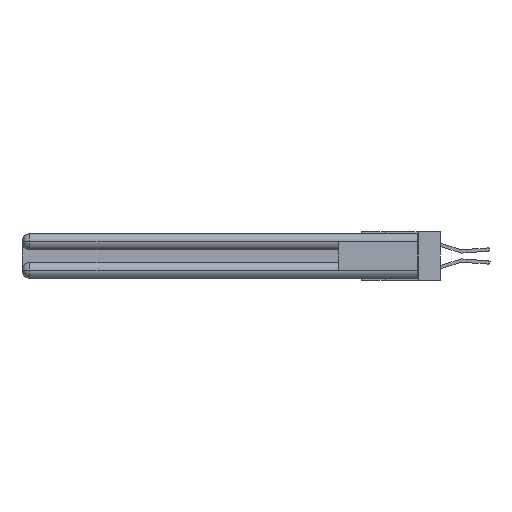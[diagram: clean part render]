
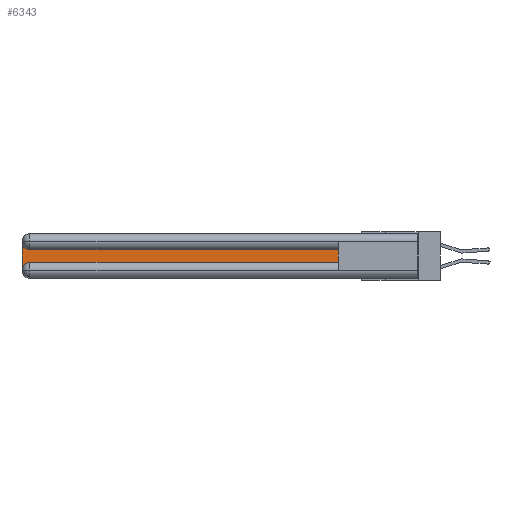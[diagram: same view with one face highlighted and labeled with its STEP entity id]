
A CAD part, left-side view. The second image highlights one B-rep face of the part: STEP entity #6343.
In plain terms, the highlighted planar face has unit normal (-1, 0, 0).
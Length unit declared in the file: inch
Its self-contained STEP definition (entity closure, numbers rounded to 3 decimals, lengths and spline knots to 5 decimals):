
#704 = ORIENTED_EDGE ( 'NONE', *, *, #27883, .T. ) ;
#1953 = LINE ( 'NONE', #17784, #20460 ) ;
#1994 = EDGE_CURVE ( 'NONE', #14123, #4935, #2353, .T. ) ;
#2238 = CARTESIAN_POINT ( 'NONE',  ( 0.075, 0.6, -0.2175 ) ) ;
#2353 = LINE ( 'NONE', #14998, #34311 ) ;
#3078 = CARTESIAN_POINT ( 'NONE',  ( 0.075, 3., -0.0625 ) ) ;
#3487 = CARTESIAN_POINT ( 'NONE',  ( 0.075, 0.6, -0.2175 ) ) ;
#4935 = VERTEX_POINT ( 'NONE', #10187 ) ;
#4954 = CARTESIAN_POINT ( 'NONE',  ( 0.075, 3., -0.2775 ) ) ;
#6296 = EDGE_CURVE ( 'NONE', #18946, #32020, #17619, .T. ) ;
#6343 = ADVANCED_FACE ( 'NONE', ( #10034 ), #30828, .F. ) ;
#6376 = CIRCLE ( 'NONE', #26609, 0.06 ) ;
#6933 = ORIENTED_EDGE ( 'NONE', *, *, #1994, .T. ) ;
#6968 = DIRECTION ( 'NONE',  ( 0., 0., -1. ) ) ;
#7288 = CARTESIAN_POINT ( 'NONE',  ( 0.075, 2.94, -0.0625 ) ) ;
#7335 = EDGE_CURVE ( 'NONE', #19390, #12281, #23789, .T. ) ;
#8816 = VECTOR ( 'NONE', #33448, 39.37008 ) ;
#9538 = CARTESIAN_POINT ( 'NONE',  ( 0.075, 3., -0.1225 ) ) ;
#10034 = FACE_OUTER_BOUND ( 'NONE', #21886, .T. ) ;
#10187 = CARTESIAN_POINT ( 'NONE',  ( 0.075, 2.94, -0.1225 ) ) ;
#10805 = EDGE_CURVE ( 'NONE', #4935, #19390, #6376, .T. ) ;
#12281 = VERTEX_POINT ( 'NONE', #4954 ) ;
#12984 = DIRECTION ( 'NONE',  ( 1., 0., 0. ) ) ;
#13157 = ORIENTED_EDGE ( 'NONE', *, *, #7335, .T. ) ;
#13812 = EDGE_CURVE ( 'NONE', #12281, #18946, #27131, .T. ) ;
#14123 = VERTEX_POINT ( 'NONE', #29299 ) ;
#14532 = CARTESIAN_POINT ( 'NONE',  ( 0.075, 3., -0.2175 ) ) ;
#14755 = DIRECTION ( 'NONE',  ( 1., 0., 0. ) ) ;
#14998 = CARTESIAN_POINT ( 'NONE',  ( 0.075, 0.6, -0.1225 ) ) ;
#16537 = CARTESIAN_POINT ( 'NONE',  ( 0.075, 2.94, -0.2175 ) ) ;
#17619 = LINE ( 'NONE', #3487, #8816 ) ;
#17784 = CARTESIAN_POINT ( 'NONE',  ( 0.075, 0.6, -0.2175 ) ) ;
#18233 = ORIENTED_EDGE ( 'NONE', *, *, #10805, .T. ) ;
#18946 = VERTEX_POINT ( 'NONE', #16537 ) ;
#19094 = ORIENTED_EDGE ( 'NONE', *, *, #6296, .T. ) ;
#19390 = VERTEX_POINT ( 'NONE', #3078 ) ;
#20384 = DIRECTION ( 'NONE',  ( 0., 1., 0. ) ) ;
#20460 = VECTOR ( 'NONE', #31300, 39.37008 ) ;
#21886 = EDGE_LOOP ( 'NONE', ( #6933, #18233, #13157, #29632, #19094, #704 ) ) ;
#23303 = DIRECTION ( 'NONE',  ( 0., 0., -1. ) ) ;
#23789 = LINE ( 'NONE', #14532, #28465 ) ;
#23885 = AXIS2_PLACEMENT_3D ( 'NONE', #31888, #12984, #23303 ) ;
#26090 = DIRECTION ( 'NONE',  ( 0., 0., -1. ) ) ;
#26609 = AXIS2_PLACEMENT_3D ( 'NONE', #7288, #33727, #28557 ) ;
#27131 = CIRCLE ( 'NONE', #23885, 0.06 ) ;
#27825 = AXIS2_PLACEMENT_3D ( 'NONE', #9538, #14755, #26090 ) ;
#27883 = EDGE_CURVE ( 'NONE', #32020, #14123, #1953, .T. ) ;
#28465 = VECTOR ( 'NONE', #6968, 39.37008 ) ;
#28557 = DIRECTION ( 'NONE',  ( 0., 0., -1. ) ) ;
#29299 = CARTESIAN_POINT ( 'NONE',  ( 0.075, 0.6, -0.1225 ) ) ;
#29632 = ORIENTED_EDGE ( 'NONE', *, *, #13812, .T. ) ;
#30828 = PLANE ( 'NONE',  #27825 ) ;
#31300 = DIRECTION ( 'NONE',  ( 0., 0., 1. ) ) ;
#31888 = CARTESIAN_POINT ( 'NONE',  ( 0.075, 2.94, -0.2775 ) ) ;
#32020 = VERTEX_POINT ( 'NONE', #2238 ) ;
#33448 = DIRECTION ( 'NONE',  ( 0., -1., 0. ) ) ;
#33727 = DIRECTION ( 'NONE',  ( 1., 0., 0. ) ) ;
#34311 = VECTOR ( 'NONE', #20384, 39.37008 ) ;
